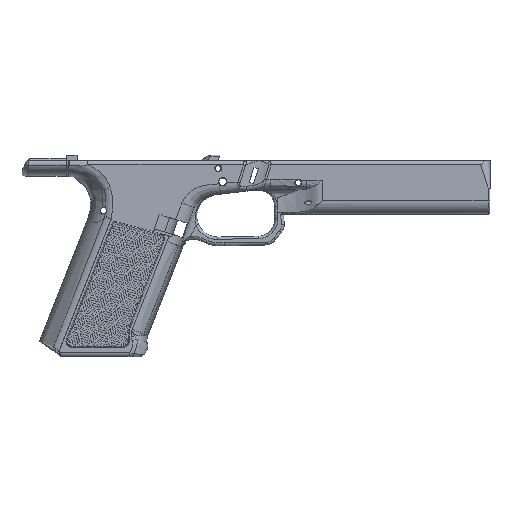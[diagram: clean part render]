
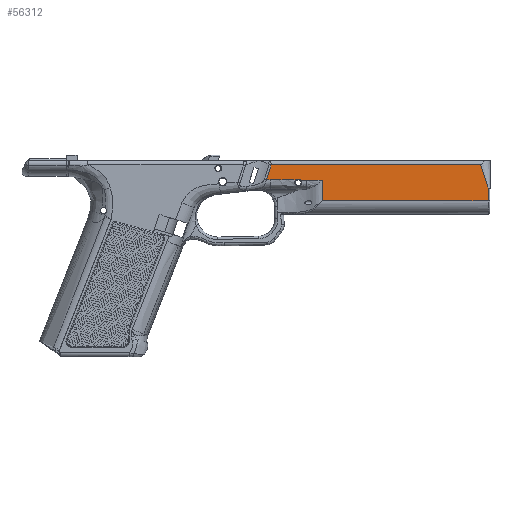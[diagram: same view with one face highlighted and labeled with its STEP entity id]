
A CAD part, top view. The second image highlights one B-rep face of the part: STEP entity #56312.
In plain terms, the highlighted planar face has unit normal (0, 0, 1).
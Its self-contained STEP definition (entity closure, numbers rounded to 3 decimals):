
#3759=CIRCLE('',#59611,5675.358);
#3760=CIRCLE('',#59612,1.799);
#3761=CIRCLE('',#59613,1.8);
#3762=CIRCLE('',#59614,5539.236);
#4422=B_SPLINE_CURVE_WITH_KNOTS('',3,(#72915,#72916,#72917,#72918),
 .UNSPECIFIED.,.F.,.F.,(4,4),(0.,1.),.UNSPECIFIED.);
#4423=B_SPLINE_CURVE_WITH_KNOTS('',3,(#72922,#72923,#72924,#72925,#72926,
#72927),.UNSPECIFIED.,.F.,.F.,(4,2,4),(0.,0.,0.),
 .UNSPECIFIED.);
#4424=B_SPLINE_CURVE_WITH_KNOTS('',3,(#72937,#72938,#72939,#72940),
 .UNSPECIFIED.,.F.,.F.,(4,4),(-0.001,0.),.UNSPECIFIED.);
#5152=FACE_OUTER_BOUND('',#8404,.T.);
#8404=EDGE_LOOP('',(#37329,#37330,#37331,#37332,#37333,#37334,#37335,#37336,
#37337,#37338,#37339,#37340,#37341,#37342,#37343));
#11865=LINE('',#72501,#17212);
#11871=LINE('',#72534,#17218);
#11878=LINE('',#72558,#17225);
#11908=LINE('',#72745,#17255);
#11929=LINE('',#72880,#17276);
#11936=LINE('',#72913,#17283);
#11937=LINE('',#72935,#17284);
#11938=LINE('',#72941,#17285);
#17212=VECTOR('',#62078,10.);
#17218=VECTOR('',#62100,10.);
#17225=VECTOR('',#62115,10.524);
#17255=VECTOR('',#62161,10.);
#17276=VECTOR('',#62200,10.);
#17283=VECTOR('',#62221,1000.);
#17284=VECTOR('',#62230,10.);
#17285=VECTOR('',#62231,10.);
#22697=VERTEX_POINT('',#72493);
#22699=VERTEX_POINT('',#72499);
#22708=VERTEX_POINT('',#72532);
#22715=VERTEX_POINT('',#72551);
#22762=VERTEX_POINT('',#72744);
#22792=VERTEX_POINT('',#72844);
#22803=VERTEX_POINT('',#72912);
#22804=VERTEX_POINT('',#72914);
#22805=VERTEX_POINT('',#72919);
#22806=VERTEX_POINT('',#72921);
#22807=VERTEX_POINT('',#72928);
#22808=VERTEX_POINT('',#72930);
#22809=VERTEX_POINT('',#72932);
#22810=VERTEX_POINT('',#72934);
#22811=VERTEX_POINT('',#72936);
#28410=EDGE_CURVE('',#22699,#22697,#11865,.T.);
#28422=EDGE_CURVE('',#22708,#22699,#11871,.T.);
#28432=EDGE_CURVE('',#22715,#22708,#11878,.T.);
#28482=EDGE_CURVE('',#22697,#22762,#11908,.T.);
#28516=EDGE_CURVE('',#22792,#22715,#11929,.T.);
#28529=EDGE_CURVE('',#22792,#22803,#11936,.T.);
#28530=EDGE_CURVE('',#22803,#22804,#4422,.T.);
#28531=EDGE_CURVE('',#22804,#22805,#3759,.T.);
#28532=EDGE_CURVE('',#22806,#22805,#4423,.T.);
#28533=EDGE_CURVE('',#22807,#22806,#3760,.T.);
#28534=EDGE_CURVE('',#22808,#22807,#3761,.T.);
#28535=EDGE_CURVE('',#22808,#22809,#3762,.T.);
#28536=EDGE_CURVE('',#22809,#22810,#11937,.T.);
#28537=EDGE_CURVE('',#22811,#22810,#4424,.T.);
#28538=EDGE_CURVE('',#22762,#22811,#11938,.T.);
#37329=ORIENTED_EDGE('',*,*,#28422,.F.);
#37330=ORIENTED_EDGE('',*,*,#28432,.F.);
#37331=ORIENTED_EDGE('',*,*,#28516,.F.);
#37332=ORIENTED_EDGE('',*,*,#28529,.T.);
#37333=ORIENTED_EDGE('',*,*,#28530,.T.);
#37334=ORIENTED_EDGE('',*,*,#28531,.T.);
#37335=ORIENTED_EDGE('',*,*,#28532,.F.);
#37336=ORIENTED_EDGE('',*,*,#28533,.F.);
#37337=ORIENTED_EDGE('',*,*,#28534,.F.);
#37338=ORIENTED_EDGE('',*,*,#28535,.T.);
#37339=ORIENTED_EDGE('',*,*,#28536,.T.);
#37340=ORIENTED_EDGE('',*,*,#28537,.F.);
#37341=ORIENTED_EDGE('',*,*,#28538,.F.);
#37342=ORIENTED_EDGE('',*,*,#28482,.F.);
#37343=ORIENTED_EDGE('',*,*,#28410,.F.);
#54651=PLANE('',#59610);
#56312=ADVANCED_FACE('',(#5152),#54651,.T.);
#59610=AXIS2_PLACEMENT_3D('',#72911,#62219,#62220);
#59611=AXIS2_PLACEMENT_3D('',#72920,#62222,#62223);
#59612=AXIS2_PLACEMENT_3D('',#72929,#62224,#62225);
#59613=AXIS2_PLACEMENT_3D('',#72931,#62226,#62227);
#59614=AXIS2_PLACEMENT_3D('',#72933,#62228,#62229);
#62078=DIRECTION('',(0.,-1.,0.));
#62100=DIRECTION('',(-1.,0.,0.));
#62115=DIRECTION('',(0.312,-0.95,0.));
#62161=DIRECTION('',(-1.,0.,0.));
#62200=DIRECTION('',(1.,0.,0.));
#62219=DIRECTION('center_axis',(0.,0.,1.));
#62220=DIRECTION('ref_axis',(1.,0.,0.));
#62221=DIRECTION('',(-0.301,-0.954,0.));
#62222=DIRECTION('center_axis',(0.,0.,
1.));
#62223=DIRECTION('ref_axis',(-0.012,-1.,0.));
#62224=DIRECTION('center_axis',(0.,0.,
1.));
#62225=DIRECTION('ref_axis',(-0.635,0.772,0.));
#62226=DIRECTION('center_axis',(0.,0.,1.));
#62227=DIRECTION('ref_axis',(1.,0.,0.));
#62228=DIRECTION('center_axis',(0.,0.,1.));
#62229=DIRECTION('ref_axis',(-0.011,-1.,0.));
#62230=DIRECTION('',(1.,0.,0.));
#62231=DIRECTION('',(0.,1.,0.));
#72493=CARTESIAN_POINT('',(122.908,-22.675,14.4));
#72499=CARTESIAN_POINT('',(122.908,-15.847,14.4));
#72501=CARTESIAN_POINT('',(122.908,-7.794,14.4));
#72532=CARTESIAN_POINT('',(122.918,-15.847,14.4));
#72534=CARTESIAN_POINT('',(11.959,-15.847,14.4));
#72551=CARTESIAN_POINT('',(118.918,-3.65,14.4));
#72558=CARTESIAN_POINT('',(120.509,-8.5,14.4));
#72744=CARTESIAN_POINT('',(35.221,-22.675,14.4));
#72745=CARTESIAN_POINT('',(11.959,-22.675,14.4));
#72844=CARTESIAN_POINT('',(8.203,-3.65,14.4));
#72880=CARTESIAN_POINT('',(8.203,-3.65,14.4));
#72911=CARTESIAN_POINT('Origin',(-100.,0.,14.4));
#72912=CARTESIAN_POINT('',(5.742,-11.454,14.4));
#72913=CARTESIAN_POINT('',(8.203,-3.65,14.4));
#72914=CARTESIAN_POINT('',(7.789,-11.434,14.4));
#72915=CARTESIAN_POINT('Ctrl Pts',(5.742,-11.454,14.4));
#72916=CARTESIAN_POINT('Ctrl Pts',(6.436,-11.44,14.4));
#72917=CARTESIAN_POINT('Ctrl Pts',(7.119,-11.434,14.4));
#72918=CARTESIAN_POINT('Ctrl Pts',(7.789,-11.434,14.4));
#72919=CARTESIAN_POINT('',(21.454,-11.612,14.4));
#72920=CARTESIAN_POINT('Origin',(88.398,5663.351,13.628));
#72921=CARTESIAN_POINT('',(21.457,-11.61,14.4));
#72922=CARTESIAN_POINT('Ctrl Pts',(21.457,-11.61,14.4));
#72923=CARTESIAN_POINT('Ctrl Pts',(21.456,-11.61,14.4));
#72924=CARTESIAN_POINT('Ctrl Pts',(21.456,-11.61,14.4));
#72925=CARTESIAN_POINT('Ctrl Pts',(21.455,-11.611,14.4));
#72926=CARTESIAN_POINT('Ctrl Pts',(21.454,-11.612,14.4));
#72927=CARTESIAN_POINT('Ctrl Pts',(21.454,-11.612,14.4));
#72928=CARTESIAN_POINT('',(21.905,-11.34,14.4));
#72929=CARTESIAN_POINT('Origin',(22.599,-12.999,14.4));
#72930=CARTESIAN_POINT('',(23.775,-11.637,14.4));
#72931=CARTESIAN_POINT('Origin',(22.6,-13.,14.4));
#72932=CARTESIAN_POINT('',(27.,-11.675,14.4));
#72933=CARTESIAN_POINT('Origin',(86.772,5527.239,14.4));
#72934=CARTESIAN_POINT('',(35.213,-11.675,14.4));
#72935=CARTESIAN_POINT('',(27.,-11.675,14.4));
#72936=CARTESIAN_POINT('',(35.221,-11.674,14.4));
#72937=CARTESIAN_POINT('Ctrl Pts',(35.221,-11.674,14.4));
#72938=CARTESIAN_POINT('Ctrl Pts',(35.218,-11.674,14.4));
#72939=CARTESIAN_POINT('Ctrl Pts',(35.215,-11.675,14.4));
#72940=CARTESIAN_POINT('Ctrl Pts',(35.213,-11.675,14.4));
#72941=CARTESIAN_POINT('',(35.221,-11.675,14.4));
